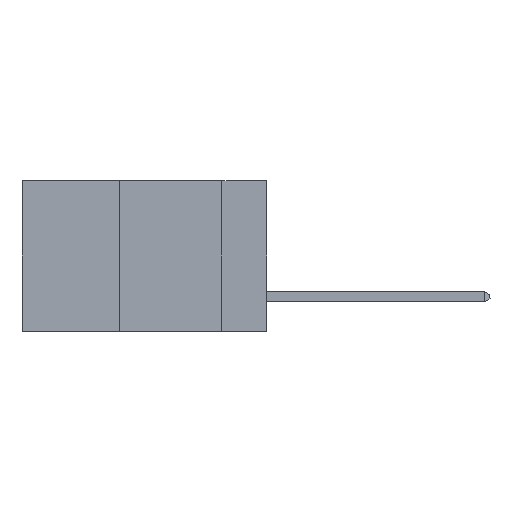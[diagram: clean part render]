
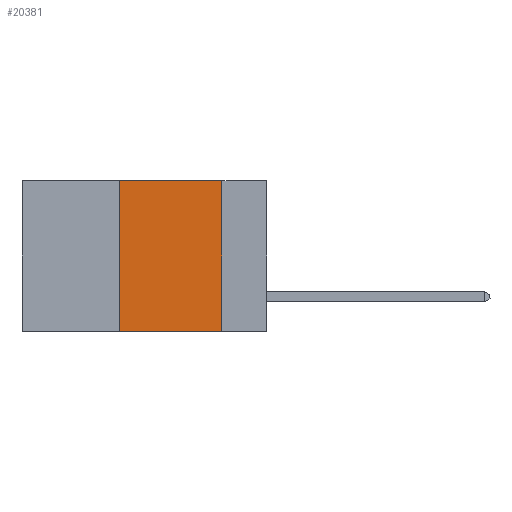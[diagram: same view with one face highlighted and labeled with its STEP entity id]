
A CAD part, left-side view. The second image highlights one B-rep face of the part: STEP entity #20381.
In plain terms, the highlighted planar face has unit normal (-1, 0, 0).
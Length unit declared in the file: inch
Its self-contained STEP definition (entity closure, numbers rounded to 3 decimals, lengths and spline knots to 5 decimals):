
#74 = ORIENTED_EDGE ( 'NONE', *, *, #21921, .F. ) ;
#1610 = ORIENTED_EDGE ( 'NONE', *, *, #28134, .F. ) ;
#2391 = DIRECTION ( 'NONE',  ( 0., 0., 1. ) ) ;
#3268 = VECTOR ( 'NONE', #24720, 39.37008 ) ;
#3618 = VECTOR ( 'NONE', #2391, 39.37008 ) ;
#6444 = PLANE ( 'NONE',  #27980 ) ;
#8883 = DIRECTION ( 'NONE',  ( 0., 0., -1. ) ) ;
#10114 = LINE ( 'NONE', #14658, #3618 ) ;
#11040 = FACE_OUTER_BOUND ( 'NONE', #17424, .T. ) ;
#11144 = CARTESIAN_POINT ( 'NONE',  ( 0., 0.36, -0.37 ) ) ;
#13649 = DIRECTION ( 'NONE',  ( 0., -1., 0. ) ) ;
#14658 = CARTESIAN_POINT ( 'NONE',  ( 0., 0.36, 0. ) ) ;
#14705 = ORIENTED_EDGE ( 'NONE', *, *, #15356, .F. ) ;
#15356 = EDGE_CURVE ( 'NONE', #17827, #26125, #10114, .T. ) ;
#16274 = CARTESIAN_POINT ( 'NONE',  ( 0., 0.36, 0. ) ) ;
#17123 = LINE ( 'NONE', #29629, #3268 ) ;
#17424 = EDGE_LOOP ( 'NONE', ( #74, #1610, #14705, #22766 ) ) ;
#17827 = VERTEX_POINT ( 'NONE', #11144 ) ;
#20364 = VECTOR ( 'NONE', #13649, 39.37008 ) ;
#20381 = ADVANCED_FACE ( 'NONE', ( #11040 ), #6444, .F. ) ;
#21204 = CARTESIAN_POINT ( 'NONE',  ( 0., 0.6, 0. ) ) ;
#21894 = LINE ( 'NONE', #25818, #20364 ) ;
#21921 = EDGE_CURVE ( 'NONE', #29991, #24955, #17123, .T. ) ;
#22072 = CARTESIAN_POINT ( 'NONE',  ( 0., 0.6, 0. ) ) ;
#22766 = ORIENTED_EDGE ( 'NONE', *, *, #29216, .T. ) ;
#23591 = CARTESIAN_POINT ( 'NONE',  ( 0., 0.11, -0.37 ) ) ;
#23642 = DIRECTION ( 'NONE',  ( 1., 0., 0. ) ) ;
#23863 = LINE ( 'NONE', #22072, #29564 ) ;
#24493 = DIRECTION ( 'NONE',  ( 0., -1., 0. ) ) ;
#24720 = DIRECTION ( 'NONE',  ( 0., 0., -1. ) ) ;
#24955 = VERTEX_POINT ( 'NONE', #23591 ) ;
#25818 = CARTESIAN_POINT ( 'NONE',  ( 0., 0.6, -0.37 ) ) ;
#26125 = VERTEX_POINT ( 'NONE', #16274 ) ;
#27148 = CARTESIAN_POINT ( 'NONE',  ( 0., 0.11, 0. ) ) ;
#27980 = AXIS2_PLACEMENT_3D ( 'NONE', #21204, #23642, #8883 ) ;
#28134 = EDGE_CURVE ( 'NONE', #26125, #29991, #23863, .T. ) ;
#29216 = EDGE_CURVE ( 'NONE', #17827, #24955, #21894, .T. ) ;
#29564 = VECTOR ( 'NONE', #24493, 39.37008 ) ;
#29629 = CARTESIAN_POINT ( 'NONE',  ( 0., 0.11, 0. ) ) ;
#29991 = VERTEX_POINT ( 'NONE', #27148 ) ;
